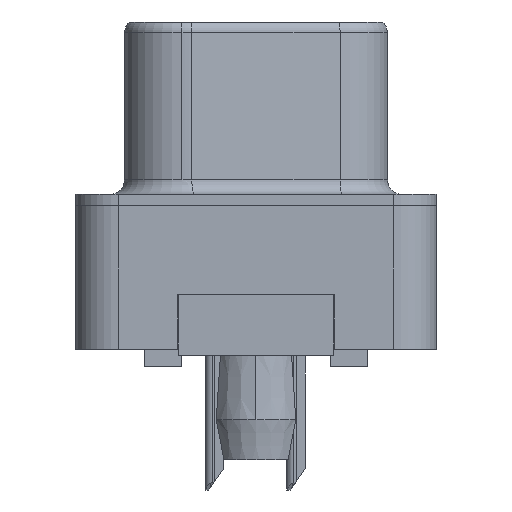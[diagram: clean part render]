
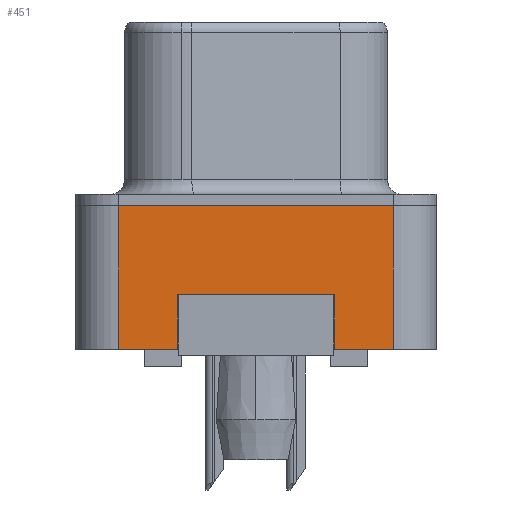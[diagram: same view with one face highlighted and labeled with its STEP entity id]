
A CAD part, left-side view. The second image highlights one B-rep face of the part: STEP entity #451.
In plain terms, the highlighted planar face has unit normal (-1, 0, 0).
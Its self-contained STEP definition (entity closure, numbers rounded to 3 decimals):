
#259 = VERTEX_POINT ( 'NONE', #20521 ) ;
#299 = AXIS2_PLACEMENT_3D ( 'NONE', #12506, #16967, #19171 ) ;
#451 = ADVANCED_FACE ( 'NONE', ( #26101 ), #8224, .T. ) ;
#664 = VECTOR ( 'NONE', #1526, 1000. ) ;
#1264 = DIRECTION ( 'NONE',  ( 0., 0., -1. ) ) ;
#1436 = CARTESIAN_POINT ( 'NONE',  ( -2.91, 2.75, -5. ) ) ;
#1525 = ORIENTED_EDGE ( 'NONE', *, *, #7281, .T. ) ;
#1526 = DIRECTION ( 'NONE',  ( 0., 0., 1. ) ) ;
#1852 = VECTOR ( 'NONE', #13892, 1000. ) ;
#2355 = VECTOR ( 'NONE', #17453, 1000. ) ;
#3160 = CARTESIAN_POINT ( 'NONE',  ( -2.91, -4.775, 0. ) ) ;
#3743 = LINE ( 'NONE', #12762, #664 ) ;
#4192 = CARTESIAN_POINT ( 'NONE',  ( -2.91, 2.75, -3.1 ) ) ;
#4339 = LINE ( 'NONE', #11279, #16037 ) ;
#4401 = ORIENTED_EDGE ( 'NONE', *, *, #12441, .F. ) ;
#4474 = DIRECTION ( 'NONE',  ( 0., 0., -1. ) ) ;
#4610 = VERTEX_POINT ( 'NONE', #19539 ) ;
#4706 = EDGE_CURVE ( 'NONE', #25788, #17722, #3743, .T. ) ;
#5033 = CARTESIAN_POINT ( 'NONE',  ( -2.91, -4.775, -5. ) ) ;
#5828 = LINE ( 'NONE', #10126, #9741 ) ;
#6331 = ORIENTED_EDGE ( 'NONE', *, *, #7521, .F. ) ;
#7220 = EDGE_CURVE ( 'NONE', #4610, #15101, #8924, .T. ) ;
#7281 = EDGE_CURVE ( 'NONE', #28976, #25788, #4339, .T. ) ;
#7521 = EDGE_CURVE ( 'NONE', #27846, #19132, #19076, .T. ) ;
#7655 = ORIENTED_EDGE ( 'NONE', *, *, #9312, .F. ) ;
#8224 = PLANE ( 'NONE',  #299 ) ;
#8695 = CARTESIAN_POINT ( 'NONE',  ( -2.91, 2.75, -3.1 ) ) ;
#8795 = VECTOR ( 'NONE', #26878, 1000. ) ;
#8924 = LINE ( 'NONE', #4192, #9894 ) ;
#9312 = EDGE_CURVE ( 'NONE', #259, #4610, #20238, .T. ) ;
#9476 = LINE ( 'NONE', #5033, #1852 ) ;
#9741 = VECTOR ( 'NONE', #1264, 1000. ) ;
#9894 = VECTOR ( 'NONE', #4474, 1000. ) ;
#10126 = CARTESIAN_POINT ( 'NONE',  ( -2.91, -2.75, -3.1 ) ) ;
#10368 = ORIENTED_EDGE ( 'NONE', *, *, #19088, .T. ) ;
#11279 = CARTESIAN_POINT ( 'NONE',  ( -2.91, -4.775, -5. ) ) ;
#12072 = VECTOR ( 'NONE', #18967, 1000. ) ;
#12441 = EDGE_CURVE ( 'NONE', #19132, #17722, #23134, .T. ) ;
#12506 = CARTESIAN_POINT ( 'NONE',  ( -2.91, -4.775, -5. ) ) ;
#12762 = CARTESIAN_POINT ( 'NONE',  ( -2.91, -4.775, -5. ) ) ;
#13209 = DIRECTION ( 'NONE',  ( 0., -1., 0. ) ) ;
#13448 = CARTESIAN_POINT ( 'NONE',  ( -2.91, 4.775, -5. ) ) ;
#13530 = EDGE_LOOP ( 'NONE', ( #10368, #1525, #25078, #4401, #6331, #22964, #28997, #7655 ) ) ;
#13892 = DIRECTION ( 'NONE',  ( 0., -1., 0. ) ) ;
#13973 = CARTESIAN_POINT ( 'NONE',  ( -2.91, -4.775, -5. ) ) ;
#15101 = VERTEX_POINT ( 'NONE', #1436 ) ;
#15888 = CARTESIAN_POINT ( 'NONE',  ( -2.91, 4.775, 0. ) ) ;
#16037 = VECTOR ( 'NONE', #13209, 1000. ) ;
#16967 = DIRECTION ( 'NONE',  ( -1., 0., 0. ) ) ;
#17453 = DIRECTION ( 'NONE',  ( 0., 0., 1. ) ) ;
#17722 = VERTEX_POINT ( 'NONE', #21724 ) ;
#18967 = DIRECTION ( 'NONE',  ( 0., -1., 0. ) ) ;
#19076 = LINE ( 'NONE', #23795, #2355 ) ;
#19088 = EDGE_CURVE ( 'NONE', #259, #28976, #5828, .T. ) ;
#19132 = VERTEX_POINT ( 'NONE', #15888 ) ;
#19171 = DIRECTION ( 'NONE',  ( 0., 0., 1. ) ) ;
#19539 = CARTESIAN_POINT ( 'NONE',  ( -2.91, 2.75, -3.1 ) ) ;
#20238 = LINE ( 'NONE', #8695, #8795 ) ;
#20521 = CARTESIAN_POINT ( 'NONE',  ( -2.91, -2.75, -3.1 ) ) ;
#21724 = CARTESIAN_POINT ( 'NONE',  ( -2.91, -4.775, 0. ) ) ;
#22964 = ORIENTED_EDGE ( 'NONE', *, *, #23701, .T. ) ;
#23134 = LINE ( 'NONE', #3160, #12072 ) ;
#23701 = EDGE_CURVE ( 'NONE', #27846, #15101, #9476, .T. ) ;
#23795 = CARTESIAN_POINT ( 'NONE',  ( -2.91, 4.775, -5. ) ) ;
#25078 = ORIENTED_EDGE ( 'NONE', *, *, #4706, .T. ) ;
#25788 = VERTEX_POINT ( 'NONE', #13973 ) ;
#26101 = FACE_OUTER_BOUND ( 'NONE', #13530, .T. ) ;
#26878 = DIRECTION ( 'NONE',  ( 0., 1., 0. ) ) ;
#27846 = VERTEX_POINT ( 'NONE', #13448 ) ;
#28511 = CARTESIAN_POINT ( 'NONE',  ( -2.91, -2.75, -5. ) ) ;
#28976 = VERTEX_POINT ( 'NONE', #28511 ) ;
#28997 = ORIENTED_EDGE ( 'NONE', *, *, #7220, .F. ) ;
